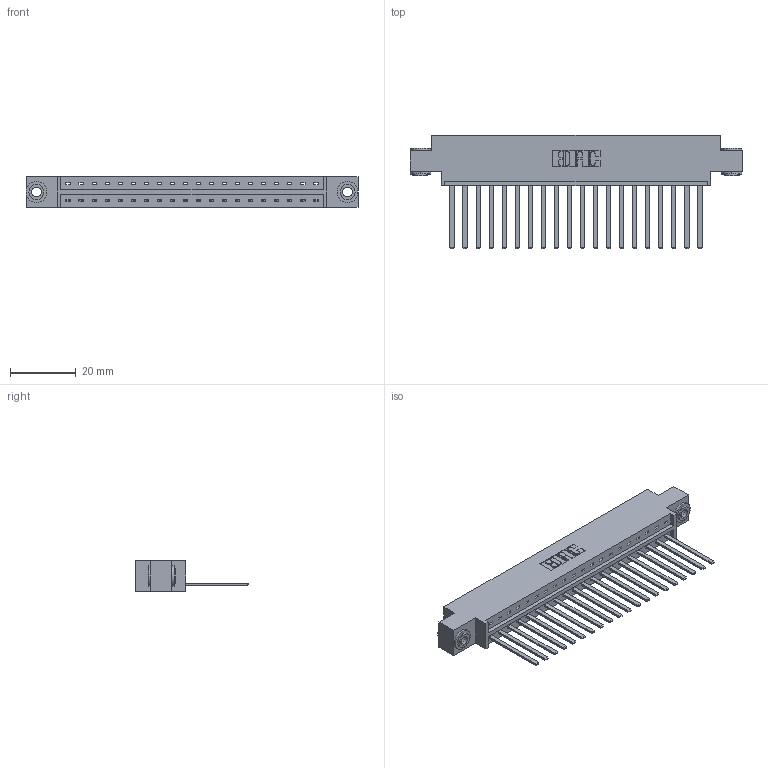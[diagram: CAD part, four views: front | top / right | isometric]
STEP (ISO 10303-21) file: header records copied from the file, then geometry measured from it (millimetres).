
FILE_DESCRIPTION (( 'STEP AP203' ), '1' );
FILE_NAME ('833-020-544-603.STEP', '2020-06-01T13:33:15', ( '' ), ( '' ), 'SwSTEP 2.0', 'SolidWorks 2020', '' );
FILE_SCHEMA (( 'CONFIG_CONTROL_DESIGN' ));
Length unit declared in the file: inch
Products named in the file (4): 833 Part_Offset - .156 Dia - TH; 345-292-001_345-293-144; 833-020-544-603; 345-250-002_345-250-002-102
Assembly tree (23 placements, depth 2):
  833-020-544-603
    833 Part_Offset - .156 Dia - TH
    345-292-001_345-293-144  x20
    345-250-002_345-250-002-102  x2
Bounding box: 100.79 x 34.3 x 9.4 mm (x, y, z)
Volume: 9976.1 mm3; surface area: 11828.7 mm2
Topology: 23 solids, 23 shells, 1196 faces, 3559 edges, 2342 vertices
Faces by surface type: plane 844, cylinder 344, cone 8
Entity records: 15670 total; most frequent: CARTESIAN_POINT 2685, ORIENTED_EDGE 2634, DIRECTION 2339, EDGE_CURVE 1317, LINE 1169, VECTOR 1169, VERTEX_POINT 874, AXIS2_PLACEMENT_3D 585
